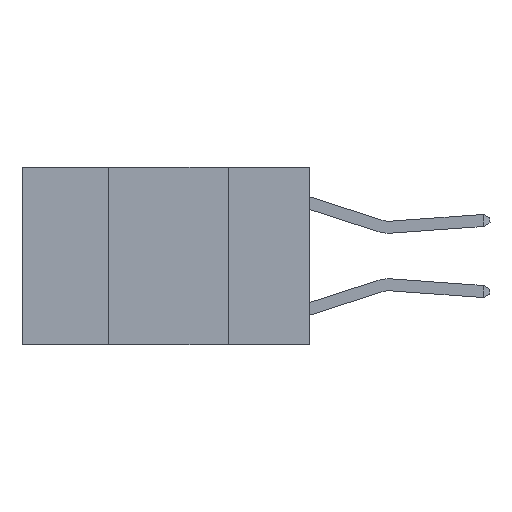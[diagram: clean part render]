
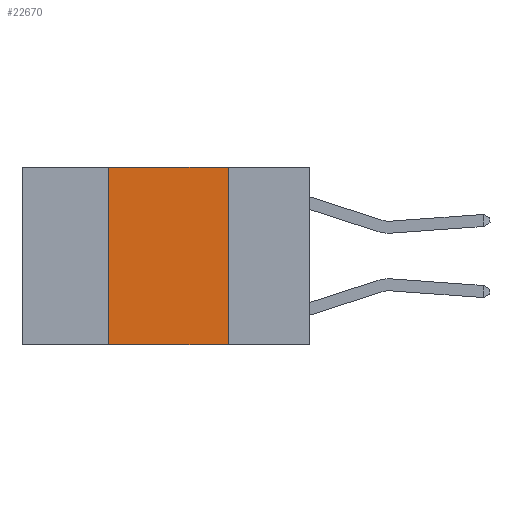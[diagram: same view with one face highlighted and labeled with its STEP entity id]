
A CAD part, left-side view. The second image highlights one B-rep face of the part: STEP entity #22670.
In plain terms, the highlighted planar face has unit normal (-1, 0, 0).
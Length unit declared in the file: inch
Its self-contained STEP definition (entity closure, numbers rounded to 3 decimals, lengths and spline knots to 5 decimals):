
#337 = EDGE_CURVE ( 'NONE', #15571, #16199, #3320, .T. ) ;
#580 = DIRECTION ( 'NONE',  ( 0., -1., 0. ) ) ;
#872 = CARTESIAN_POINT ( 'NONE',  ( 0., 0.17, 0. ) ) ;
#1358 = LINE ( 'NONE', #11513, #6378 ) ;
#3139 = ORIENTED_EDGE ( 'NONE', *, *, #9278, .F. ) ;
#3318 = CARTESIAN_POINT ( 'NONE',  ( 0., 0.42, 0. ) ) ;
#3320 = LINE ( 'NONE', #3318, #15800 ) ;
#3665 = EDGE_CURVE ( 'NONE', #5382, #3959, #7005, .T. ) ;
#3959 = VERTEX_POINT ( 'NONE', #15109 ) ;
#5382 = VERTEX_POINT ( 'NONE', #18827 ) ;
#5730 = VECTOR ( 'NONE', #580, 39.37008 ) ;
#6378 = VECTOR ( 'NONE', #22502, 39.37008 ) ;
#6554 = DIRECTION ( 'NONE',  ( 0., 0., -1. ) ) ;
#6615 = CARTESIAN_POINT ( 'NONE',  ( 0., 0.42, 0. ) ) ;
#7005 = LINE ( 'NONE', #872, #21159 ) ;
#7257 = EDGE_CURVE ( 'NONE', #15571, #3959, #1358, .T. ) ;
#7274 = CARTESIAN_POINT ( 'NONE',  ( 0., 0.6, 0. ) ) ;
#8052 = AXIS2_PLACEMENT_3D ( 'NONE', #7274, #20170, #9112 ) ;
#9112 = DIRECTION ( 'NONE',  ( 0., 0., -1. ) ) ;
#9237 = ORIENTED_EDGE ( 'NONE', *, *, #7257, .T. ) ;
#9278 = EDGE_CURVE ( 'NONE', #16199, #5382, #20456, .T. ) ;
#10693 = ORIENTED_EDGE ( 'NONE', *, *, #3665, .F. ) ;
#11513 = CARTESIAN_POINT ( 'NONE',  ( 0., 0.6, -0.37 ) ) ;
#12321 = CARTESIAN_POINT ( 'NONE',  ( 0., 0.42, -0.37 ) ) ;
#13598 = ORIENTED_EDGE ( 'NONE', *, *, #337, .F. ) ;
#13615 = CARTESIAN_POINT ( 'NONE',  ( 0., 0.6, 0. ) ) ;
#15109 = CARTESIAN_POINT ( 'NONE',  ( 0., 0.17, -0.37 ) ) ;
#15571 = VERTEX_POINT ( 'NONE', #12321 ) ;
#15800 = VECTOR ( 'NONE', #19912, 39.37008 ) ;
#16199 = VERTEX_POINT ( 'NONE', #6615 ) ;
#17508 = EDGE_LOOP ( 'NONE', ( #10693, #3139, #13598, #9237 ) ) ;
#18315 = PLANE ( 'NONE',  #8052 ) ;
#18827 = CARTESIAN_POINT ( 'NONE',  ( 0., 0.17, 0. ) ) ;
#19912 = DIRECTION ( 'NONE',  ( 0., 0., 1. ) ) ;
#20170 = DIRECTION ( 'NONE',  ( 1., 0., 0. ) ) ;
#20456 = LINE ( 'NONE', #13615, #5730 ) ;
#21032 = FACE_OUTER_BOUND ( 'NONE', #17508, .T. ) ;
#21159 = VECTOR ( 'NONE', #6554, 39.37008 ) ;
#22502 = DIRECTION ( 'NONE',  ( 0., -1., 0. ) ) ;
#22670 = ADVANCED_FACE ( 'NONE', ( #21032 ), #18315, .F. ) ;
